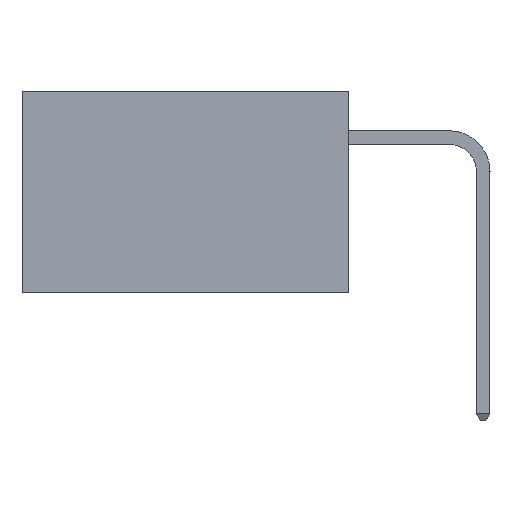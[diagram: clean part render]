
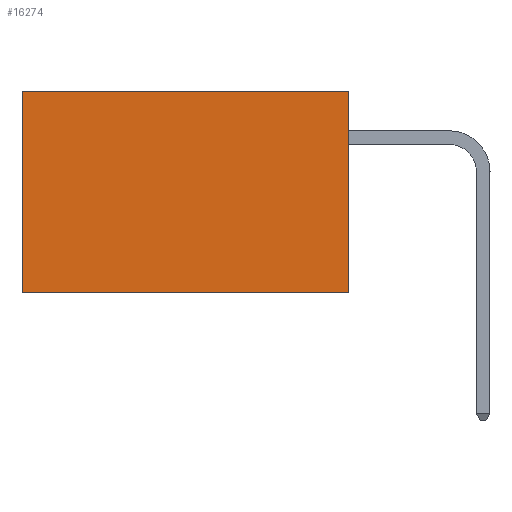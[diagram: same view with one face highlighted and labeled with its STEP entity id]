
A CAD part, left-side view. The second image highlights one B-rep face of the part: STEP entity #16274.
In plain terms, the highlighted planar face has unit normal (-1, 0, 0).
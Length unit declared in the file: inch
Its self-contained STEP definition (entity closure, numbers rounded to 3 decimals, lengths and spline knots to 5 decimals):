
#484 = DIRECTION ( 'NONE',  ( 1., 0., 0. ) ) ;
#2241 = EDGE_CURVE ( 'NONE', #18945, #3729, #31682, .T. ) ;
#2934 = ORIENTED_EDGE ( 'NONE', *, *, #7630, .T. ) ;
#3279 = DIRECTION ( 'NONE',  ( 0., 0., -1. ) ) ;
#3729 = VERTEX_POINT ( 'NONE', #20707 ) ;
#4121 = LINE ( 'NONE', #21166, #8547 ) ;
#4834 = DIRECTION ( 'NONE',  ( 0., 0., -1. ) ) ;
#5369 = CARTESIAN_POINT ( 'NONE',  ( 0.2875, 0., 0. ) ) ;
#6949 = ORIENTED_EDGE ( 'NONE', *, *, #2241, .F. ) ;
#7630 = EDGE_CURVE ( 'NONE', #35930, #36958, #4121, .T. ) ;
#8547 = VECTOR ( 'NONE', #36460, 39.37008 ) ;
#9815 = EDGE_LOOP ( 'NONE', ( #11992, #6949, #32279, #2934 ) ) ;
#11266 = AXIS2_PLACEMENT_3D ( 'NONE', #36647, #484, #35119 ) ;
#11992 = ORIENTED_EDGE ( 'NONE', *, *, #32680, .T. ) ;
#14798 = DIRECTION ( 'NONE',  ( 0., 1., 0. ) ) ;
#15857 = LINE ( 'NONE', #23530, #25011 ) ;
#16274 = ADVANCED_FACE ( 'NONE', ( #20381 ), #29662, .F. ) ;
#18622 = VECTOR ( 'NONE', #14798, 39.37008 ) ;
#18945 = VERTEX_POINT ( 'NONE', #28477 ) ;
#18991 = CARTESIAN_POINT ( 'NONE',  ( 0.2875, 0.6, 0. ) ) ;
#20330 = CARTESIAN_POINT ( 'NONE',  ( 0.2875, 0., -0.37 ) ) ;
#20381 = FACE_OUTER_BOUND ( 'NONE', #9815, .T. ) ;
#20707 = CARTESIAN_POINT ( 'NONE',  ( 0.2875, 0.6, -0.37 ) ) ;
#21166 = CARTESIAN_POINT ( 'NONE',  ( 0.2875, 0., 0. ) ) ;
#23530 = CARTESIAN_POINT ( 'NONE',  ( 0.2875, 0., 0. ) ) ;
#24387 = EDGE_CURVE ( 'NONE', #35930, #18945, #15857, .T. ) ;
#25011 = VECTOR ( 'NONE', #4834, 39.37008 ) ;
#27517 = VECTOR ( 'NONE', #3279, 39.37008 ) ;
#28477 = CARTESIAN_POINT ( 'NONE',  ( 0.2875, 0., -0.37 ) ) ;
#29662 = PLANE ( 'NONE',  #11266 ) ;
#30938 = LINE ( 'NONE', #18991, #27517 ) ;
#31682 = LINE ( 'NONE', #20330, #18622 ) ;
#32279 = ORIENTED_EDGE ( 'NONE', *, *, #24387, .F. ) ;
#32680 = EDGE_CURVE ( 'NONE', #36958, #3729, #30938, .T. ) ;
#34946 = CARTESIAN_POINT ( 'NONE',  ( 0.2875, 0.6, 0. ) ) ;
#35119 = DIRECTION ( 'NONE',  ( 0., 0., -1. ) ) ;
#35930 = VERTEX_POINT ( 'NONE', #5369 ) ;
#36460 = DIRECTION ( 'NONE',  ( 0., 1., 0. ) ) ;
#36647 = CARTESIAN_POINT ( 'NONE',  ( 0.2875, 0., 0. ) ) ;
#36958 = VERTEX_POINT ( 'NONE', #34946 ) ;
